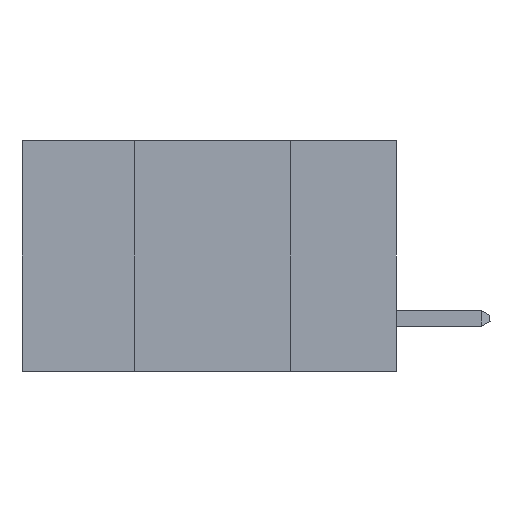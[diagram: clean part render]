
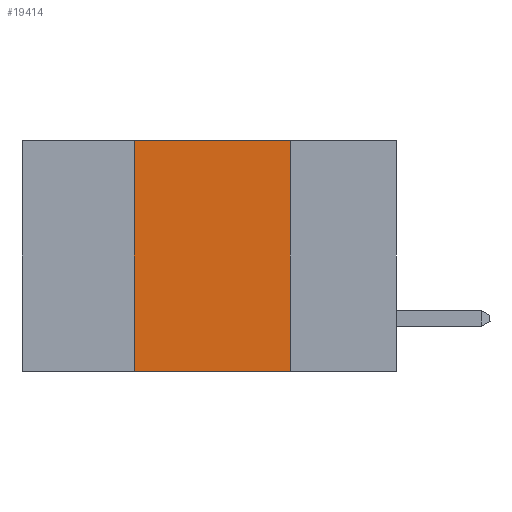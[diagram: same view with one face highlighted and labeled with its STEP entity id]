
A CAD part, left-side view. The second image highlights one B-rep face of the part: STEP entity #19414.
In plain terms, the highlighted planar face has unit normal (-1, 0, 0).
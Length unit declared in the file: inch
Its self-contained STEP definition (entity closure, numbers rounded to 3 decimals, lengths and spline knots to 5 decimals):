
#12 = CARTESIAN_POINT ( 'NONE',  ( 0., 0.17, 0. ) ) ;
#283 = CARTESIAN_POINT ( 'NONE',  ( 0., 0.42, -0.37 ) ) ;
#396 = VECTOR ( 'NONE', #12646, 39.37008 ) ;
#1510 = LINE ( 'NONE', #14326, #396 ) ;
#1799 = VERTEX_POINT ( 'NONE', #18383 ) ;
#1846 = ORIENTED_EDGE ( 'NONE', *, *, #17781, .F. ) ;
#2423 = VERTEX_POINT ( 'NONE', #3834 ) ;
#2724 = ORIENTED_EDGE ( 'NONE', *, *, #9626, .T. ) ;
#2971 = VECTOR ( 'NONE', #10267, 39.37008 ) ;
#3834 = CARTESIAN_POINT ( 'NONE',  ( 0., 0.17, -0.37 ) ) ;
#4904 = CARTESIAN_POINT ( 'NONE',  ( 0., 0.17, 0. ) ) ;
#5067 = VECTOR ( 'NONE', #17588, 39.37008 ) ;
#5165 = ORIENTED_EDGE ( 'NONE', *, *, #18488, .F. ) ;
#5690 = DIRECTION ( 'NONE',  ( 1., 0., 0. ) ) ;
#6531 = FACE_OUTER_BOUND ( 'NONE', #8237, .T. ) ;
#8237 = EDGE_LOOP ( 'NONE', ( #5165, #19705, #1846, #2724 ) ) ;
#8373 = CARTESIAN_POINT ( 'NONE',  ( 0., 0.42, 0. ) ) ;
#9626 = EDGE_CURVE ( 'NONE', #10669, #2423, #1510, .T. ) ;
#10092 = VERTEX_POINT ( 'NONE', #12 ) ;
#10267 = DIRECTION ( 'NONE',  ( 0., 0., 1. ) ) ;
#10669 = VERTEX_POINT ( 'NONE', #283 ) ;
#12646 = DIRECTION ( 'NONE',  ( 0., -1., 0. ) ) ;
#13070 = LINE ( 'NONE', #8373, #2971 ) ;
#14326 = CARTESIAN_POINT ( 'NONE',  ( 0., 0.6, -0.37 ) ) ;
#15320 = AXIS2_PLACEMENT_3D ( 'NONE', #21318, #5690, #18006 ) ;
#15586 = DIRECTION ( 'NONE',  ( 0., 0., -1. ) ) ;
#15880 = CARTESIAN_POINT ( 'NONE',  ( 0., 0.6, 0. ) ) ;
#16303 = PLANE ( 'NONE',  #15320 ) ;
#17588 = DIRECTION ( 'NONE',  ( 0., -1., 0. ) ) ;
#17781 = EDGE_CURVE ( 'NONE', #10669, #1799, #13070, .T. ) ;
#18006 = DIRECTION ( 'NONE',  ( 0., 0., -1. ) ) ;
#18383 = CARTESIAN_POINT ( 'NONE',  ( 0., 0.42, 0. ) ) ;
#18488 = EDGE_CURVE ( 'NONE', #10092, #2423, #19738, .T. ) ;
#19100 = LINE ( 'NONE', #15880, #5067 ) ;
#19210 = VECTOR ( 'NONE', #15586, 39.37008 ) ;
#19414 = ADVANCED_FACE ( 'NONE', ( #6531 ), #16303, .F. ) ;
#19705 = ORIENTED_EDGE ( 'NONE', *, *, #22736, .F. ) ;
#19738 = LINE ( 'NONE', #4904, #19210 ) ;
#21318 = CARTESIAN_POINT ( 'NONE',  ( 0., 0.6, 0. ) ) ;
#22736 = EDGE_CURVE ( 'NONE', #1799, #10092, #19100, .T. ) ;
